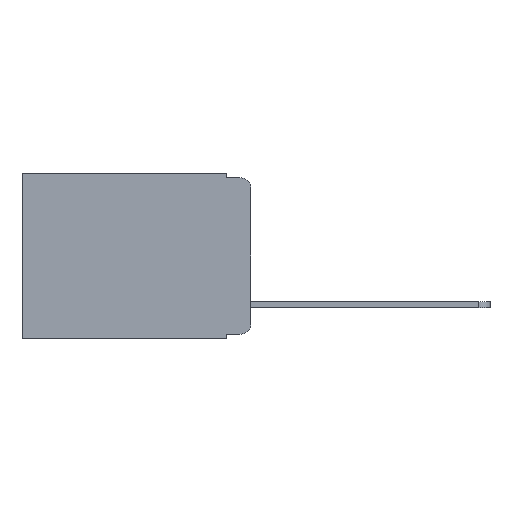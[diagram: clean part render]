
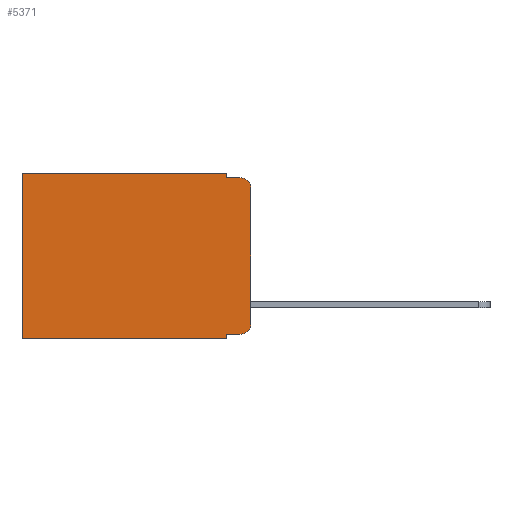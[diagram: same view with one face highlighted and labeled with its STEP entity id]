
A CAD part, left-side view. The second image highlights one B-rep face of the part: STEP entity #5371.
In plain terms, the highlighted planar face has unit normal (-1, 0, 0).
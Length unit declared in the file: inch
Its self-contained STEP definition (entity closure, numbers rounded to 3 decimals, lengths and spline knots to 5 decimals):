
#197 = ORIENTED_EDGE ( 'NONE', *, *, #18301, .T. ) ;
#378 = DIRECTION ( 'NONE',  ( -1., 0., 0. ) ) ;
#450 = EDGE_CURVE ( 'NONE', #14705, #6786, #9280, .T. ) ;
#1006 = VERTEX_POINT ( 'NONE', #9490 ) ;
#1057 = EDGE_CURVE ( 'NONE', #1006, #14705, #8104, .T. ) ;
#1330 = ORIENTED_EDGE ( 'NONE', *, *, #2508, .T. ) ;
#1384 = VERTEX_POINT ( 'NONE', #9742 ) ;
#1626 = CARTESIAN_POINT ( 'NONE',  ( 0.298, 0., -0.03 ) ) ;
#1827 = AXIS2_PLACEMENT_3D ( 'NONE', #2805, #8525, #13114 ) ;
#1934 = ORIENTED_EDGE ( 'NONE', *, *, #11797, .T. ) ;
#2410 = CIRCLE ( 'NONE', #1827, 0.02 ) ;
#2412 = CARTESIAN_POINT ( 'NONE',  ( 0.298, 0.051, -0.333 ) ) ;
#2508 = EDGE_CURVE ( 'NONE', #10137, #11716, #6719, .T. ) ;
#2805 = CARTESIAN_POINT ( 'NONE',  ( 0.298, 0.02, -0.03 ) ) ;
#2929 = EDGE_CURVE ( 'NONE', #11154, #1384, #4239, .T. ) ;
#3116 = AXIS2_PLACEMENT_3D ( 'NONE', #10521, #7657, #15047 ) ;
#3172 = DIRECTION ( 'NONE',  ( 0., 0., -1. ) ) ;
#3316 = EDGE_CURVE ( 'NONE', #10137, #17838, #3789, .T. ) ;
#3362 = CARTESIAN_POINT ( 'NONE',  ( 0.298, 0.473, 0. ) ) ;
#3572 = AXIS2_PLACEMENT_3D ( 'NONE', #4800, #378, #16554 ) ;
#3608 = ORIENTED_EDGE ( 'NONE', *, *, #8298, .T. ) ;
#3789 = LINE ( 'NONE', #16479, #11521 ) ;
#4026 = CARTESIAN_POINT ( 'NONE',  ( 0.298, 0.051, 0. ) ) ;
#4091 = CARTESIAN_POINT ( 'NONE',  ( 0.298, 0.051, -0.01 ) ) ;
#4233 = LINE ( 'NONE', #7619, #7622 ) ;
#4239 = LINE ( 'NONE', #6564, #16028 ) ;
#4764 = CIRCLE ( 'NONE', #3572, 0.02 ) ;
#4790 = DIRECTION ( 'NONE',  ( 0., 0., -1. ) ) ;
#4800 = CARTESIAN_POINT ( 'NONE',  ( 0.298, 0.02, -0.313 ) ) ;
#4873 = CARTESIAN_POINT ( 'NONE',  ( 0.298, 0.051, -0.343 ) ) ;
#4934 = EDGE_CURVE ( 'NONE', #1006, #14448, #9162, .T. ) ;
#5331 = ORIENTED_EDGE ( 'NONE', *, *, #4934, .T. ) ;
#5371 = ADVANCED_FACE ( 'NONE', ( #17577 ), #16369, .F. ) ;
#6181 = DIRECTION ( 'NONE',  ( 0., 0., -1. ) ) ;
#6392 = CARTESIAN_POINT ( 'NONE',  ( 0.298, 0.02, -0.01 ) ) ;
#6452 = CARTESIAN_POINT ( 'NONE',  ( 0.298, 0.473, -0.343 ) ) ;
#6564 = CARTESIAN_POINT ( 'NONE',  ( 0.298, 0., 0. ) ) ;
#6719 = LINE ( 'NONE', #17054, #11066 ) ;
#6776 = VERTEX_POINT ( 'NONE', #6452 ) ;
#6786 = VERTEX_POINT ( 'NONE', #6392 ) ;
#7278 = ORIENTED_EDGE ( 'NONE', *, *, #18456, .F. ) ;
#7619 = CARTESIAN_POINT ( 'NONE',  ( 0.298, 0., -0.343 ) ) ;
#7622 = VECTOR ( 'NONE', #11977, 39.37008 ) ;
#7657 = DIRECTION ( 'NONE',  ( 1., 0., 0. ) ) ;
#8104 = LINE ( 'NONE', #4026, #16040 ) ;
#8298 = EDGE_CURVE ( 'NONE', #14448, #6776, #18791, .T. ) ;
#8525 = DIRECTION ( 'NONE',  ( -1., 0., 0. ) ) ;
#8533 = DIRECTION ( 'NONE',  ( 0., 1., 0. ) ) ;
#8539 = ORIENTED_EDGE ( 'NONE', *, *, #3316, .F. ) ;
#9162 = LINE ( 'NONE', #18785, #16193 ) ;
#9280 = LINE ( 'NONE', #4091, #17237 ) ;
#9490 = CARTESIAN_POINT ( 'NONE',  ( 0.298, 0.051, 0. ) ) ;
#9634 = CARTESIAN_POINT ( 'NONE',  ( 0.298, 0.051, -0.01 ) ) ;
#9742 = CARTESIAN_POINT ( 'NONE',  ( 0.298, 0., -0.313 ) ) ;
#9869 = DIRECTION ( 'NONE',  ( 0., -1., 0. ) ) ;
#10137 = VERTEX_POINT ( 'NONE', #2412 ) ;
#10521 = CARTESIAN_POINT ( 'NONE',  ( 0.298, 0., 0. ) ) ;
#10971 = DIRECTION ( 'NONE',  ( 0., 0., -1. ) ) ;
#11066 = VECTOR ( 'NONE', #11455, 39.37008 ) ;
#11154 = VERTEX_POINT ( 'NONE', #1626 ) ;
#11455 = DIRECTION ( 'NONE',  ( 0., -1., 0. ) ) ;
#11521 = VECTOR ( 'NONE', #4790, 39.37008 ) ;
#11716 = VERTEX_POINT ( 'NONE', #17542 ) ;
#11797 = EDGE_CURVE ( 'NONE', #11716, #1384, #4764, .T. ) ;
#11971 = VECTOR ( 'NONE', #3172, 39.37008 ) ;
#11977 = DIRECTION ( 'NONE',  ( 0., 1., 0. ) ) ;
#12835 = EDGE_LOOP ( 'NONE', ( #13319, #197, #18276, #16960, #5331, #3608, #7278, #8539, #1330, #1934 ) ) ;
#13114 = DIRECTION ( 'NONE',  ( 0., 0., -1. ) ) ;
#13319 = ORIENTED_EDGE ( 'NONE', *, *, #2929, .F. ) ;
#14448 = VERTEX_POINT ( 'NONE', #18320 ) ;
#14705 = VERTEX_POINT ( 'NONE', #9634 ) ;
#15047 = DIRECTION ( 'NONE',  ( 0., 0., -1. ) ) ;
#16028 = VECTOR ( 'NONE', #10971, 39.37008 ) ;
#16040 = VECTOR ( 'NONE', #6181, 39.37008 ) ;
#16193 = VECTOR ( 'NONE', #8533, 39.37008 ) ;
#16369 = PLANE ( 'NONE',  #3116 ) ;
#16479 = CARTESIAN_POINT ( 'NONE',  ( 0.298, 0.051, 0. ) ) ;
#16554 = DIRECTION ( 'NONE',  ( 0., 0., -1. ) ) ;
#16960 = ORIENTED_EDGE ( 'NONE', *, *, #1057, .F. ) ;
#17054 = CARTESIAN_POINT ( 'NONE',  ( 0.298, 0.051, -0.333 ) ) ;
#17237 = VECTOR ( 'NONE', #9869, 39.37008 ) ;
#17542 = CARTESIAN_POINT ( 'NONE',  ( 0.298, 0.02, -0.333 ) ) ;
#17577 = FACE_OUTER_BOUND ( 'NONE', #12835, .T. ) ;
#17838 = VERTEX_POINT ( 'NONE', #4873 ) ;
#18276 = ORIENTED_EDGE ( 'NONE', *, *, #450, .F. ) ;
#18301 = EDGE_CURVE ( 'NONE', #11154, #6786, #2410, .T. ) ;
#18320 = CARTESIAN_POINT ( 'NONE',  ( 0.298, 0.473, 0. ) ) ;
#18456 = EDGE_CURVE ( 'NONE', #17838, #6776, #4233, .T. ) ;
#18785 = CARTESIAN_POINT ( 'NONE',  ( 0.298, 0., 0. ) ) ;
#18791 = LINE ( 'NONE', #3362, #11971 ) ;
